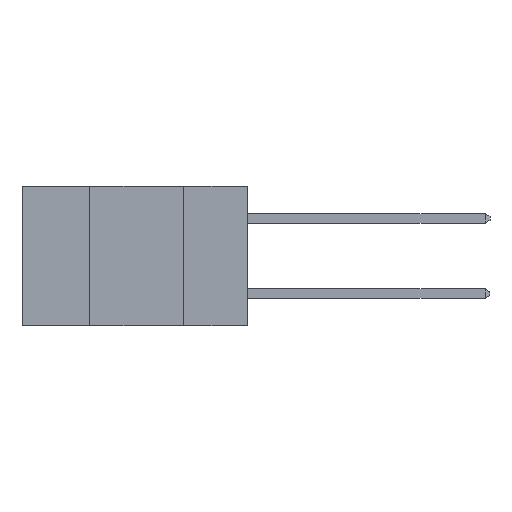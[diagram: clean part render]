
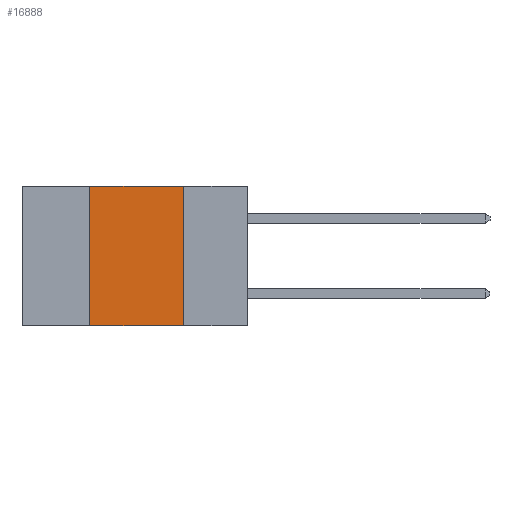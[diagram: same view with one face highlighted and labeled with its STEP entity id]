
A CAD part, left-side view. The second image highlights one B-rep face of the part: STEP entity #16888.
In plain terms, the highlighted planar face has unit normal (-1, 0, 0).
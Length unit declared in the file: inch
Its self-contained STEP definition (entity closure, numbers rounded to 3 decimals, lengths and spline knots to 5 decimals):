
#796 = DIRECTION ( 'NONE',  ( 0., 0., -1. ) ) ;
#1271 = CARTESIAN_POINT ( 'NONE',  ( 0., 0.17, -0.37 ) ) ;
#1967 = ORIENTED_EDGE ( 'NONE', *, *, #13809, .F. ) ;
#2071 = AXIS2_PLACEMENT_3D ( 'NONE', #17244, #9235, #796 ) ;
#2246 = CARTESIAN_POINT ( 'NONE',  ( 0., 0.42, 0. ) ) ;
#2254 = CARTESIAN_POINT ( 'NONE',  ( 0., 0.6, -0.37 ) ) ;
#2419 = ORIENTED_EDGE ( 'NONE', *, *, #8728, .T. ) ;
#3926 = LINE ( 'NONE', #15268, #6797 ) ;
#4540 = CARTESIAN_POINT ( 'NONE',  ( 0., 0.17, 0. ) ) ;
#4738 = VECTOR ( 'NONE', #10631, 39.37008 ) ;
#5270 = LINE ( 'NONE', #12704, #11720 ) ;
#5662 = EDGE_CURVE ( 'NONE', #7199, #15039, #5270, .T. ) ;
#6243 = FACE_OUTER_BOUND ( 'NONE', #10748, .T. ) ;
#6797 = VECTOR ( 'NONE', #16576, 39.37008 ) ;
#7109 = LINE ( 'NONE', #2254, #4738 ) ;
#7199 = VERTEX_POINT ( 'NONE', #4540 ) ;
#7553 = DIRECTION ( 'NONE',  ( 0., 0., 1. ) ) ;
#7852 = PLANE ( 'NONE',  #2071 ) ;
#8728 = EDGE_CURVE ( 'NONE', #14011, #15039, #7109, .T. ) ;
#8911 = CARTESIAN_POINT ( 'NONE',  ( 0., 0.42, 0. ) ) ;
#9235 = DIRECTION ( 'NONE',  ( 1., 0., 0. ) ) ;
#9318 = LINE ( 'NONE', #8911, #12507 ) ;
#10631 = DIRECTION ( 'NONE',  ( 0., -1., 0. ) ) ;
#10748 = EDGE_LOOP ( 'NONE', ( #16156, #1967, #16573, #2419 ) ) ;
#11720 = VECTOR ( 'NONE', #17698, 39.37008 ) ;
#12507 = VECTOR ( 'NONE', #7553, 39.37008 ) ;
#12704 = CARTESIAN_POINT ( 'NONE',  ( 0., 0.17, 0. ) ) ;
#13809 = EDGE_CURVE ( 'NONE', #16201, #7199, #3926, .T. ) ;
#14011 = VERTEX_POINT ( 'NONE', #15649 ) ;
#15039 = VERTEX_POINT ( 'NONE', #1271 ) ;
#15268 = CARTESIAN_POINT ( 'NONE',  ( 0., 0.6, 0. ) ) ;
#15403 = EDGE_CURVE ( 'NONE', #14011, #16201, #9318, .T. ) ;
#15649 = CARTESIAN_POINT ( 'NONE',  ( 0., 0.42, -0.37 ) ) ;
#16156 = ORIENTED_EDGE ( 'NONE', *, *, #5662, .F. ) ;
#16201 = VERTEX_POINT ( 'NONE', #2246 ) ;
#16573 = ORIENTED_EDGE ( 'NONE', *, *, #15403, .F. ) ;
#16576 = DIRECTION ( 'NONE',  ( 0., -1., 0. ) ) ;
#16888 = ADVANCED_FACE ( 'NONE', ( #6243 ), #7852, .F. ) ;
#17244 = CARTESIAN_POINT ( 'NONE',  ( 0., 0.6, 0. ) ) ;
#17698 = DIRECTION ( 'NONE',  ( 0., 0., -1. ) ) ;
